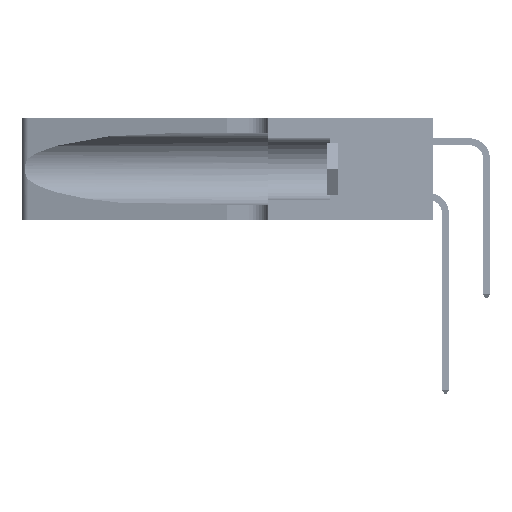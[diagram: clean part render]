
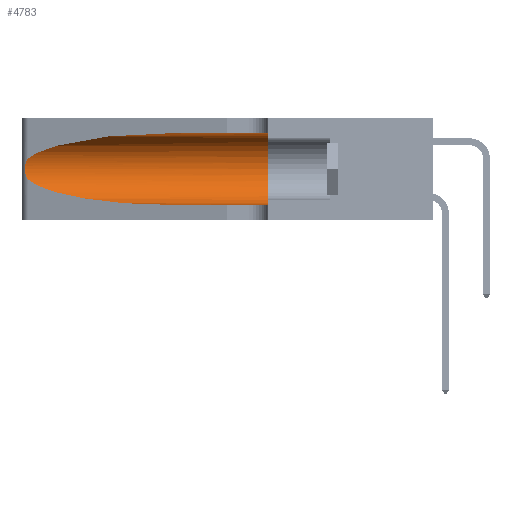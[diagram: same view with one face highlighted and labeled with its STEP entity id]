
A CAD part, left-side view. The second image highlights one B-rep face of the part: STEP entity #4783.
In plain terms, the highlighted cylindrical face has radius 3.308 mm (diameter 6.617 mm), a partial arc.
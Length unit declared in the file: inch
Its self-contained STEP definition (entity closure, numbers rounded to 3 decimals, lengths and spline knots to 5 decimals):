
#292 = EDGE_CURVE ( 'NONE', #10597, #34741, #25184, .T. ) ;
#671 = EDGE_CURVE ( 'NONE', #32201, #6938, #35419, .T. ) ;
#1201 = CARTESIAN_POINT ( 'NONE',  ( 0.18966, 0.96281, 0.31525 ) ) ;
#1441 = LINE ( 'NONE', #48076, #40206 ) ;
#1447 = CARTESIAN_POINT ( 'NONE',  ( 0.1305, 0.72297, 0.05475 ) ) ;
#1828 = EDGE_CURVE ( 'NONE', #5198, #6938, #24840, .T. ) ;
#2086 = ORIENTED_EDGE ( 'NONE', *, *, #292, .T. ) ;
#2456 = CARTESIAN_POINT ( 'NONE',  ( 0.25639, 1.23184, 0.21858 ) ) ;
#2958 = DIRECTION ( 'NONE',  ( 0., -1., 0. ) ) ;
#4470 = ORIENTED_EDGE ( 'NONE', *, *, #5058, .T. ) ;
#4783 = ADVANCED_FACE ( 'NONE', ( #11188 ), #29937, .F. ) ;
#5058 = EDGE_CURVE ( 'NONE', #7691, #5198, #16575, .T. ) ;
#5198 = VERTEX_POINT ( 'NONE', #30805 ) ;
#6181 = CARTESIAN_POINT ( 'NONE',  ( 0.25487, 1.22718, 0.14631 ) ) ;
#6337 = CARTESIAN_POINT ( 'NONE',  ( 0.25854, 1.2359, 0.20912 ) ) ;
#6469 = ORIENTED_EDGE ( 'NONE', *, *, #671, .F. ) ;
#6938 = VERTEX_POINT ( 'NONE', #31466 ) ;
#7691 = VERTEX_POINT ( 'NONE', #6181 ) ;
#8055 = DIRECTION ( 'NONE',  ( 0., 1., 0. ) ) ;
#10171 = CARTESIAN_POINT ( 'NONE',  ( 0.26075, 1.23896, 0.19203 ) ) ;
#10597 = VERTEX_POINT ( 'NONE', #24584 ) ;
#11188 = FACE_OUTER_BOUND ( 'NONE', #18843, .T. ) ;
#12104 = ORIENTED_EDGE ( 'NONE', *, *, #21055, .F. ) ;
#13413 = CARTESIAN_POINT ( 'NONE',  ( 0.25487, 1.22718, 0.22369 ) ) ;
#14019 = CARTESIAN_POINT ( 'NONE',  ( 0.26017, 1.23833, 0.17102 ) ) ;
#15567 = CARTESIAN_POINT ( 'NONE',  ( 0.1305, 0.35, 0.31525 ) ) ;
#16575 =( BOUNDED_CURVE ( )  B_SPLINE_CURVE ( 3, ( #46331, #38913, #16688, #1447 ),
 .UNSPECIFIED., .F., .F. ) 
 B_SPLINE_CURVE_WITH_KNOTS ( ( 4, 4 ),
 ( 3.44316, 4.71239 ),
 .UNSPECIFIED. ) 
 CURVE ( )  GEOMETRIC_REPRESENTATION_ITEM ( )  RATIONAL_B_SPLINE_CURVE ( ( 1., 0.87, 0.87, 1. ) ) 
 REPRESENTATION_ITEM ( '' )  );
#16608 = CARTESIAN_POINT ( 'NONE',  ( 0.25487, 1.22718, 0.22369 ) ) ;
#16688 = CARTESIAN_POINT ( 'NONE',  ( 0.18966, 0.96281, 0.05475 ) ) ;
#17406 = DIRECTION ( 'NONE',  ( 0., 0., -1. ) ) ;
#17451 = DIRECTION ( 'NONE',  ( 0., -1., 0. ) ) ;
#17839 = CARTESIAN_POINT ( 'NONE',  ( 0.25789, 1.23486, 0.15765 ) ) ;
#18843 = EDGE_LOOP ( 'NONE', ( #2086, #29099, #4470, #21590, #6469, #12104 ) ) ;
#21055 = EDGE_CURVE ( 'NONE', #10597, #32201, #1441, .T. ) ;
#21391 = CARTESIAN_POINT ( 'NONE',  ( 0.25487, 1.22718, 0.22369 ) ) ;
#21554 = CARTESIAN_POINT ( 'NONE',  ( 0.25555, 1.22993, 0.14849 ) ) ;
#21590 = ORIENTED_EDGE ( 'NONE', *, *, #1828, .T. ) ;
#23089 = B_SPLINE_CURVE_WITH_KNOTS ( 'NONE', 3,
 ( #21391, #25120, #2456, #28881, #6337, #32583, #10171, #36293, #14019, #40044, #17839, #43753, #21554, #47454 ),
 .UNSPECIFIED., .F., .F.,
 ( 4, 2, 2, 2, 2, 2, 4 ),
 ( 0., 0.00027, 0.00053, 0.00107, 0.0016, 0.00187, 0.00214 ),
 .UNSPECIFIED. ) ;
#24584 = CARTESIAN_POINT ( 'NONE',  ( 0.1305, 0.72297, 0.31525 ) ) ;
#24840 = LINE ( 'NONE', #24893, #34710 ) ;
#24893 = CARTESIAN_POINT ( 'NONE',  ( 0.1305, 1.61858, 0.05475 ) ) ;
#25120 = CARTESIAN_POINT ( 'NONE',  ( 0.25555, 1.22994, 0.2215 ) ) ;
#25184 =( BOUNDED_CURVE ( )  B_SPLINE_CURVE ( 3, ( #38834, #1201, #42384, #16608 ),
 .UNSPECIFIED., .F., .F. ) 
 B_SPLINE_CURVE_WITH_KNOTS ( ( 4, 4 ),
 ( 1.5708, 2.84003 ),
 .UNSPECIFIED. ) 
 CURVE ( )  GEOMETRIC_REPRESENTATION_ITEM ( )  RATIONAL_B_SPLINE_CURVE ( ( 1., 0.87, 0.87, 1. ) ) 
 REPRESENTATION_ITEM ( '' )  );
#26429 = CARTESIAN_POINT ( 'NONE',  ( 0.1305, 1.61858, 0.185 ) ) ;
#28881 = CARTESIAN_POINT ( 'NONE',  ( 0.25787, 1.23484, 0.2124 ) ) ;
#29099 = ORIENTED_EDGE ( 'NONE', *, *, #44402, .T. ) ;
#29937 = CYLINDRICAL_SURFACE ( 'NONE', #32012, 0.13025 ) ;
#30547 = CARTESIAN_POINT ( 'NONE',  ( 0.1305, 0.35, 0.185 ) ) ;
#30805 = CARTESIAN_POINT ( 'NONE',  ( 0.1305, 0.72297, 0.05475 ) ) ;
#31466 = CARTESIAN_POINT ( 'NONE',  ( 0.1305, 0.35, 0.05475 ) ) ;
#32012 = AXIS2_PLACEMENT_3D ( 'NONE', #26429, #41173, #17406 ) ;
#32201 = VERTEX_POINT ( 'NONE', #15567 ) ;
#32526 = AXIS2_PLACEMENT_3D ( 'NONE', #30547, #8055, #34262 ) ;
#32583 = CARTESIAN_POINT ( 'NONE',  ( 0.26018, 1.23835, 0.19895 ) ) ;
#34262 = DIRECTION ( 'NONE',  ( 0., 0., 1. ) ) ;
#34710 = VECTOR ( 'NONE', #17451, 39.37008 ) ;
#34741 = VERTEX_POINT ( 'NONE', #13413 ) ;
#35419 = CIRCLE ( 'NONE', #32526, 0.13025 ) ;
#36293 = CARTESIAN_POINT ( 'NONE',  ( 0.26075, 1.23896, 0.178 ) ) ;
#38834 = CARTESIAN_POINT ( 'NONE',  ( 0.1305, 0.72297, 0.31525 ) ) ;
#38913 = CARTESIAN_POINT ( 'NONE',  ( 0.2373, 1.15595, 0.08982 ) ) ;
#40044 = CARTESIAN_POINT ( 'NONE',  ( 0.25856, 1.23593, 0.16098 ) ) ;
#40206 = VECTOR ( 'NONE', #2958, 39.37008 ) ;
#41173 = DIRECTION ( 'NONE',  ( 0., -1., 0. ) ) ;
#42384 = CARTESIAN_POINT ( 'NONE',  ( 0.2373, 1.15595, 0.28018 ) ) ;
#43753 = CARTESIAN_POINT ( 'NONE',  ( 0.25639, 1.23186, 0.15144 ) ) ;
#44402 = EDGE_CURVE ( 'NONE', #34741, #7691, #23089, .T. ) ;
#46331 = CARTESIAN_POINT ( 'NONE',  ( 0.25487, 1.22718, 0.14631 ) ) ;
#47454 = CARTESIAN_POINT ( 'NONE',  ( 0.25487, 1.22718, 0.14631 ) ) ;
#48076 = CARTESIAN_POINT ( 'NONE',  ( 0.1305, 1.61858, 0.31525 ) ) ;
